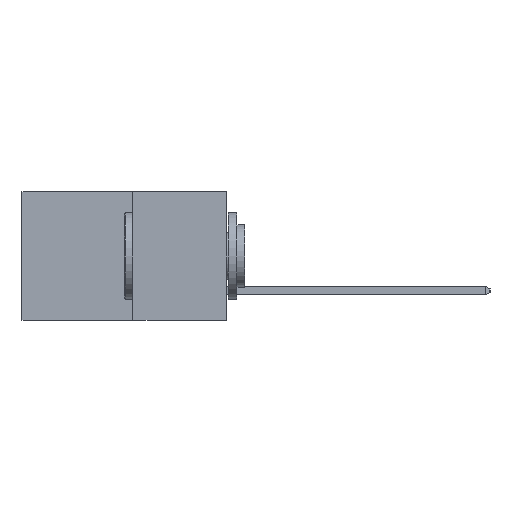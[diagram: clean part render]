
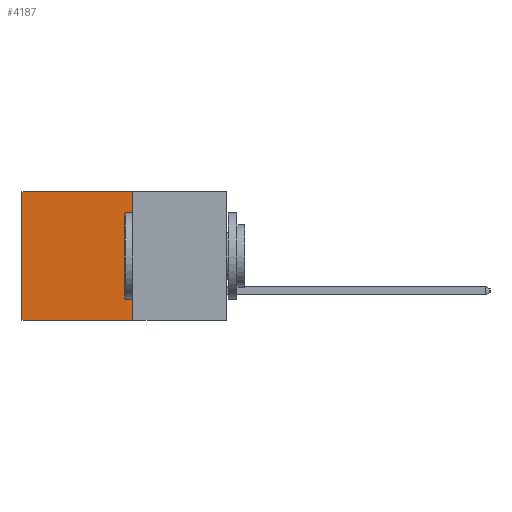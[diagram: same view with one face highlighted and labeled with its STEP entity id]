
A CAD part, left-side view. The second image highlights one B-rep face of the part: STEP entity #4187.
In plain terms, the highlighted planar face has unit normal (-1, 0, 0).
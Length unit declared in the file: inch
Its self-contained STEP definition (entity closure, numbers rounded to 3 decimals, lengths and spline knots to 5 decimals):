
#74 = VERTEX_POINT ( 'NONE', #9080 ) ;
#482 = DIRECTION ( 'NONE',  ( 0., 0., -1. ) ) ;
#538 = DIRECTION ( 'NONE',  ( 1., 0., 0. ) ) ;
#573 = ORIENTED_EDGE ( 'NONE', *, *, #8083, .T. ) ;
#1097 = PLANE ( 'NONE',  #3350 ) ;
#1114 = DIRECTION ( 'NONE',  ( 0., 0., -1. ) ) ;
#1173 = CARTESIAN_POINT ( 'NONE',  ( 0.277, 0.27, -0.37 ) ) ;
#1831 = VECTOR ( 'NONE', #1114, 39.37008 ) ;
#1925 = LINE ( 'NONE', #3108, #9358 ) ;
#2168 = CARTESIAN_POINT ( 'NONE',  ( 0.277, 0.59, 0. ) ) ;
#2366 = DIRECTION ( 'NONE',  ( 0., 0., -1. ) ) ;
#2535 = CARTESIAN_POINT ( 'NONE',  ( 0.277, 0.27, -0.37 ) ) ;
#3108 = CARTESIAN_POINT ( 'NONE',  ( 0.277, 0.27, -0.37 ) ) ;
#3189 = VERTEX_POINT ( 'NONE', #9188 ) ;
#3322 = DIRECTION ( 'NONE',  ( 0., 1., 0. ) ) ;
#3341 = CARTESIAN_POINT ( 'NONE',  ( 0.277, 0.59, -0.37 ) ) ;
#3350 = AXIS2_PLACEMENT_3D ( 'NONE', #1173, #538, #482 ) ;
#3603 = EDGE_CURVE ( 'NONE', #3189, #74, #1925, .T. ) ;
#3807 = VERTEX_POINT ( 'NONE', #5119 ) ;
#3857 = LINE ( 'NONE', #3341, #1831 ) ;
#3929 = FACE_OUTER_BOUND ( 'NONE', #5865, .T. ) ;
#4187 = ADVANCED_FACE ( 'NONE', ( #3929 ), #1097, .F. ) ;
#4542 = ORIENTED_EDGE ( 'NONE', *, *, #3603, .F. ) ;
#4814 = ORIENTED_EDGE ( 'NONE', *, *, #5595, .F. ) ;
#5033 = ORIENTED_EDGE ( 'NONE', *, *, #6487, .T. ) ;
#5113 = VECTOR ( 'NONE', #6461, 39.37008 ) ;
#5119 = CARTESIAN_POINT ( 'NONE',  ( 0.277, 0.27, 0. ) ) ;
#5580 = VECTOR ( 'NONE', #2366, 39.37008 ) ;
#5595 = EDGE_CURVE ( 'NONE', #3807, #3189, #7445, .T. ) ;
#5865 = EDGE_LOOP ( 'NONE', ( #573, #4542, #4814, #5033 ) ) ;
#6461 = DIRECTION ( 'NONE',  ( 0., 1., 0. ) ) ;
#6487 = EDGE_CURVE ( 'NONE', #3807, #7865, #8865, .T. ) ;
#6611 = CARTESIAN_POINT ( 'NONE',  ( 0.277, 0.27, 0. ) ) ;
#7445 = LINE ( 'NONE', #2535, #5580 ) ;
#7865 = VERTEX_POINT ( 'NONE', #2168 ) ;
#8083 = EDGE_CURVE ( 'NONE', #7865, #74, #3857, .T. ) ;
#8865 = LINE ( 'NONE', #6611, #5113 ) ;
#9080 = CARTESIAN_POINT ( 'NONE',  ( 0.277, 0.59, -0.37 ) ) ;
#9188 = CARTESIAN_POINT ( 'NONE',  ( 0.277, 0.27, -0.37 ) ) ;
#9358 = VECTOR ( 'NONE', #3322, 39.37008 ) ;
